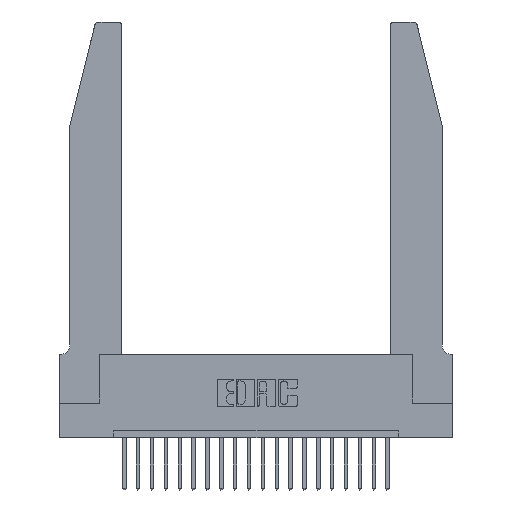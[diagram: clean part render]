
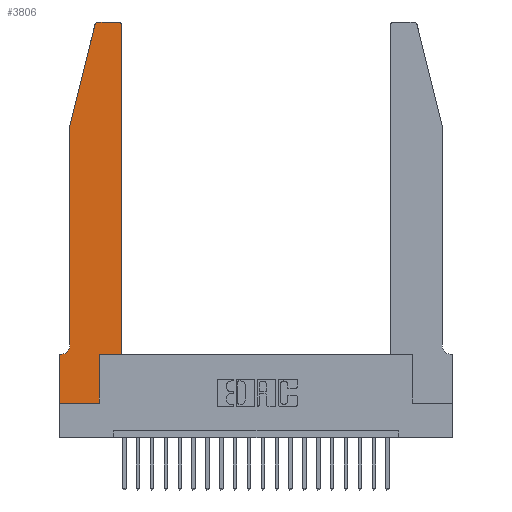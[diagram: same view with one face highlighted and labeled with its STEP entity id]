
A CAD part, top view. The second image highlights one B-rep face of the part: STEP entity #3806.
In plain terms, the highlighted planar face has unit normal (0, 0, 1).
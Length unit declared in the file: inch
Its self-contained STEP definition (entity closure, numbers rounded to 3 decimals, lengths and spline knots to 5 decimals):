
#215 = CARTESIAN_POINT ( 'NONE',  ( 0.25487, 2.72718, 0.37 ) ) ;
#293 = DIRECTION ( 'NONE',  ( 1., 0., 0. ) ) ;
#304 = CARTESIAN_POINT ( 'NONE',  ( 0.2865, 0., 0.37 ) ) ;
#507 = VECTOR ( 'NONE', #11326, 39.37008 ) ;
#1092 = ORIENTED_EDGE ( 'NONE', *, *, #16744, .T. ) ;
#1531 = DIRECTION ( 'NONE',  ( 0., 1., 0. ) ) ;
#1538 = EDGE_CURVE ( 'NONE', #16320, #9099, #9343, .T. ) ;
#1660 = EDGE_CURVE ( 'NONE', #12853, #17874, #17619, .T. ) ;
#1966 = CARTESIAN_POINT ( 'NONE',  ( 0., 0., 0.37 ) ) ;
#2555 = LINE ( 'NONE', #2561, #4197 ) ;
#2561 = CARTESIAN_POINT ( 'NONE',  ( 0., 0., 0.37 ) ) ;
#2633 = VERTEX_POINT ( 'NONE', #13954 ) ;
#3068 = VECTOR ( 'NONE', #11546, 39.37008 ) ;
#3670 = CARTESIAN_POINT ( 'NONE',  ( 0.4505, 0.35, 0.37 ) ) ;
#3806 = ADVANCED_FACE ( 'NONE', ( #5938 ), #9950, .T. ) ;
#3967 = EDGE_CURVE ( 'NONE', #9099, #14067, #10867, .T. ) ;
#4163 = DIRECTION ( 'NONE',  ( 1., 0., 0. ) ) ;
#4197 = VECTOR ( 'NONE', #20395, 39.37008 ) ;
#4210 = EDGE_CURVE ( 'NONE', #14067, #8686, #15836, .T. ) ;
#4712 = VECTOR ( 'NONE', #17570, 39.37008 ) ;
#5080 = ORIENTED_EDGE ( 'NONE', *, *, #21536, .T. ) ;
#5240 = CARTESIAN_POINT ( 'NONE',  ( 0.2865, 0.35, 0.37 ) ) ;
#5274 = EDGE_CURVE ( 'NONE', #17478, #21378, #2555, .T. ) ;
#5280 = ORIENTED_EDGE ( 'NONE', *, *, #21426, .T. ) ;
#5938 = FACE_OUTER_BOUND ( 'NONE', #18387, .T. ) ;
#5948 = VERTEX_POINT ( 'NONE', #7501 ) ;
#5955 = ORIENTED_EDGE ( 'NONE', *, *, #3967, .T. ) ;
#6062 = EDGE_CURVE ( 'NONE', #17874, #13908, #22057, .T. ) ;
#6514 = DIRECTION ( 'NONE',  ( 1., 0., 0. ) ) ;
#6687 = CARTESIAN_POINT ( 'NONE',  ( 0., 0.35, 0.37 ) ) ;
#7005 = DIRECTION ( 'NONE',  ( 0., 1., 0. ) ) ;
#7102 = CARTESIAN_POINT ( 'NONE',  ( 0.0755, 2., 0.37 ) ) ;
#7501 = CARTESIAN_POINT ( 'NONE',  ( 0.0055, 0.35, 0.37 ) ) ;
#7789 = CARTESIAN_POINT ( 'NONE',  ( 0.2605, 2.75, 0.37 ) ) ;
#8006 = VECTOR ( 'NONE', #10553, 39.37008 ) ;
#8449 = CARTESIAN_POINT ( 'NONE',  ( 0.0055, 0.42, 0.37 ) ) ;
#8686 = VERTEX_POINT ( 'NONE', #9414 ) ;
#8942 = CARTESIAN_POINT ( 'NONE',  ( 0.0755, 2., 0.37 ) ) ;
#8982 = EDGE_CURVE ( 'NONE', #8686, #17716, #11520, .T. ) ;
#9099 = VERTEX_POINT ( 'NONE', #13087 ) ;
#9343 = LINE ( 'NONE', #5240, #17632 ) ;
#9414 = CARTESIAN_POINT ( 'NONE',  ( 0.4505, 2.72, 0.37 ) ) ;
#9424 = ORIENTED_EDGE ( 'NONE', *, *, #1538, .T. ) ;
#9577 = ORIENTED_EDGE ( 'NONE', *, *, #6062, .T. ) ;
#9950 = PLANE ( 'NONE',  #10921 ) ;
#10189 = DIRECTION ( 'NONE',  ( 0., 0., 1. ) ) ;
#10553 = DIRECTION ( 'NONE',  ( -1., 0., 0. ) ) ;
#10809 = CARTESIAN_POINT ( 'NONE',  ( 0.0755, 2., 0.37 ) ) ;
#10835 = CARTESIAN_POINT ( 'NONE',  ( 0.284, 2.72, 0.37 ) ) ;
#10867 = LINE ( 'NONE', #13099, #12533 ) ;
#10921 = AXIS2_PLACEMENT_3D ( 'NONE', #20726, #10189, #6514 ) ;
#11326 = DIRECTION ( 'NONE',  ( -0.239, -0.971, 0. ) ) ;
#11520 = CIRCLE ( 'NONE', #16167, 0.03 ) ;
#11546 = DIRECTION ( 'NONE',  ( -1., 0., 0. ) ) ;
#12000 = CARTESIAN_POINT ( 'NONE',  ( 0.4505, 0.35, 0.37 ) ) ;
#12533 = VECTOR ( 'NONE', #4163, 39.37008 ) ;
#12853 = VERTEX_POINT ( 'NONE', #215 ) ;
#12931 = ORIENTED_EDGE ( 'NONE', *, *, #5274, .T. ) ;
#13087 = CARTESIAN_POINT ( 'NONE',  ( 0.2865, 0.35, 0.37 ) ) ;
#13099 = CARTESIAN_POINT ( 'NONE',  ( 0.4505, 0.35, 0.37 ) ) ;
#13908 = VERTEX_POINT ( 'NONE', #14939 ) ;
#13954 = CARTESIAN_POINT ( 'NONE',  ( 0.284, 2.75, 0.37 ) ) ;
#14067 = VERTEX_POINT ( 'NONE', #12000 ) ;
#14133 = DIRECTION ( 'NONE',  ( 1., 0., 0. ) ) ;
#14499 = ORIENTED_EDGE ( 'NONE', *, *, #1660, .T. ) ;
#14939 = CARTESIAN_POINT ( 'NONE',  ( 0.0755, 0.42, 0.37 ) ) ;
#15673 = DIRECTION ( 'NONE',  ( -1., 0., 0. ) ) ;
#15721 = CARTESIAN_POINT ( 'NONE',  ( 0.4205, 2.72, 0.37 ) ) ;
#15836 = LINE ( 'NONE', #3670, #19166 ) ;
#16167 = AXIS2_PLACEMENT_3D ( 'NONE', #15721, #19350, #22792 ) ;
#16320 = VERTEX_POINT ( 'NONE', #304 ) ;
#16454 = VECTOR ( 'NONE', #14133, 39.37008 ) ;
#16570 = ORIENTED_EDGE ( 'NONE', *, *, #8982, .T. ) ;
#16744 = EDGE_CURVE ( 'NONE', #13908, #5948, #16946, .T. ) ;
#16946 = CIRCLE ( 'NONE', #20998, 0.07 ) ;
#17269 = ORIENTED_EDGE ( 'NONE', *, *, #22678, .T. ) ;
#17422 = CARTESIAN_POINT ( 'NONE',  ( 0., 0., 0.37 ) ) ;
#17478 = VERTEX_POINT ( 'NONE', #6687 ) ;
#17570 = DIRECTION ( 'NONE',  ( 0., -1., 0. ) ) ;
#17619 = LINE ( 'NONE', #10809, #507 ) ;
#17632 = VECTOR ( 'NONE', #1531, 39.37008 ) ;
#17716 = VERTEX_POINT ( 'NONE', #18970 ) ;
#17874 = VERTEX_POINT ( 'NONE', #8942 ) ;
#17932 = DIRECTION ( 'NONE',  ( 0., 0., 1. ) ) ;
#18176 = CIRCLE ( 'NONE', #21267, 0.03 ) ;
#18387 = EDGE_LOOP ( 'NONE', ( #20370, #5080, #14499, #9577, #1092, #5280, #12931, #17269, #9424, #5955, #19832, #16570 ) ) ;
#18970 = CARTESIAN_POINT ( 'NONE',  ( 0.4205, 2.75, 0.37 ) ) ;
#19166 = VECTOR ( 'NONE', #7005, 39.37008 ) ;
#19350 = DIRECTION ( 'NONE',  ( 0., 0., 1. ) ) ;
#19832 = ORIENTED_EDGE ( 'NONE', *, *, #4210, .T. ) ;
#20370 = ORIENTED_EDGE ( 'NONE', *, *, #21133, .T. ) ;
#20395 = DIRECTION ( 'NONE',  ( 0., -1., 0. ) ) ;
#20659 = DIRECTION ( 'NONE',  ( 0., 0., -1. ) ) ;
#20726 = CARTESIAN_POINT ( 'NONE',  ( 0., 0.35, 0.37 ) ) ;
#20998 = AXIS2_PLACEMENT_3D ( 'NONE', #8449, #20659, #15673 ) ;
#21018 = CARTESIAN_POINT ( 'NONE',  ( 0.0755, 0.35, 0.37 ) ) ;
#21133 = EDGE_CURVE ( 'NONE', #17716, #2633, #21495, .T. ) ;
#21155 = LINE ( 'NONE', #1966, #16454 ) ;
#21267 = AXIS2_PLACEMENT_3D ( 'NONE', #10835, #17932, #293 ) ;
#21378 = VERTEX_POINT ( 'NONE', #17422 ) ;
#21426 = EDGE_CURVE ( 'NONE', #5948, #17478, #21756, .T. ) ;
#21495 = LINE ( 'NONE', #7789, #3068 ) ;
#21536 = EDGE_CURVE ( 'NONE', #2633, #12853, #18176, .T. ) ;
#21756 = LINE ( 'NONE', #21018, #8006 ) ;
#22057 = LINE ( 'NONE', #7102, #4712 ) ;
#22678 = EDGE_CURVE ( 'NONE', #21378, #16320, #21155, .T. ) ;
#22792 = DIRECTION ( 'NONE',  ( 1., 0., 0. ) ) ;
